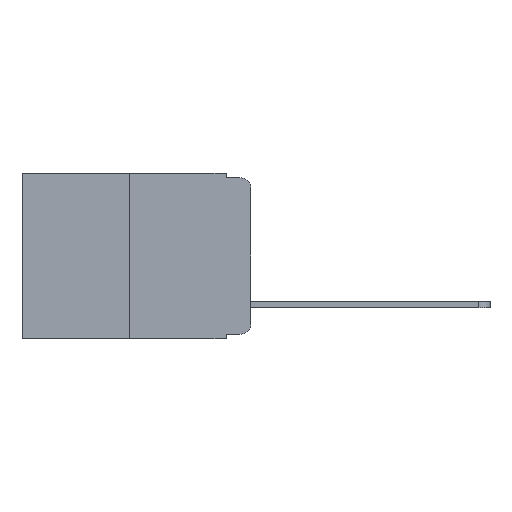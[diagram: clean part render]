
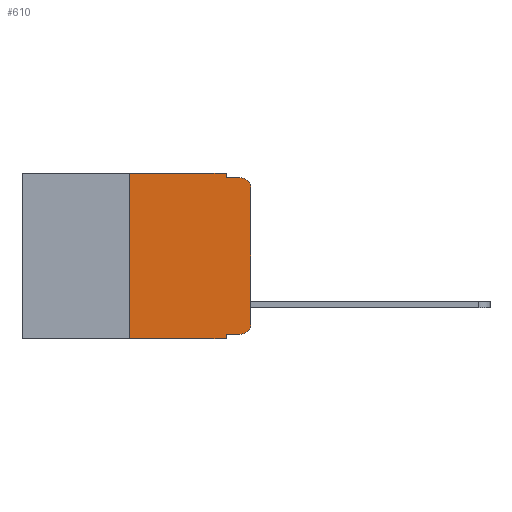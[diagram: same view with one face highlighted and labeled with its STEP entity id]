
A CAD part, left-side view. The second image highlights one B-rep face of the part: STEP entity #610.
In plain terms, the highlighted planar face has unit normal (-1, 0, 0).
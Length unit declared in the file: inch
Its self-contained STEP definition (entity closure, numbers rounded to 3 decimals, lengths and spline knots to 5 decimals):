
#143 = VERTEX_POINT ( 'NONE', #9389 ) ;
#241 = CARTESIAN_POINT ( 'NONE',  ( 0., 0.051, 0. ) ) ;
#284 = ORIENTED_EDGE ( 'NONE', *, *, #2498, .F. ) ;
#610 = ADVANCED_FACE ( 'NONE', ( #7530 ), #2642, .F. ) ;
#1050 = VERTEX_POINT ( 'NONE', #1367 ) ;
#1134 = EDGE_CURVE ( 'NONE', #5379, #143, #9879, .T. ) ;
#1167 = CARTESIAN_POINT ( 'NONE',  ( 0., 0.02, -0.03 ) ) ;
#1315 = DIRECTION ( 'NONE',  ( 0., 0., -1. ) ) ;
#1367 = CARTESIAN_POINT ( 'NONE',  ( 0., 0.051, -0.333 ) ) ;
#1408 = EDGE_CURVE ( 'NONE', #9601, #5036, #2824, .T. ) ;
#1498 = CARTESIAN_POINT ( 'NONE',  ( 0., 0., 0. ) ) ;
#1551 = EDGE_CURVE ( 'NONE', #2093, #10796, #10320, .T. ) ;
#1696 = CARTESIAN_POINT ( 'NONE',  ( 0., 0.473, 0. ) ) ;
#1870 = LINE ( 'NONE', #1498, #2463 ) ;
#1888 = VECTOR ( 'NONE', #8993, 39.37008 ) ;
#2073 = ORIENTED_EDGE ( 'NONE', *, *, #2184, .F. ) ;
#2093 = VERTEX_POINT ( 'NONE', #9987 ) ;
#2184 = EDGE_CURVE ( 'NONE', #9601, #8978, #5876, .T. ) ;
#2463 = VECTOR ( 'NONE', #3433, 39.37008 ) ;
#2498 = EDGE_CURVE ( 'NONE', #10796, #9502, #9255, .T. ) ;
#2527 = VECTOR ( 'NONE', #11309, 39.37008 ) ;
#2642 = PLANE ( 'NONE',  #5559 ) ;
#2744 = ORIENTED_EDGE ( 'NONE', *, *, #3947, .T. ) ;
#2749 = LINE ( 'NONE', #4065, #4204 ) ;
#2762 = CARTESIAN_POINT ( 'NONE',  ( 0., 0.25, -0.343 ) ) ;
#2796 = CARTESIAN_POINT ( 'NONE',  ( 0., 0.02, -0.01 ) ) ;
#2824 = LINE ( 'NONE', #5761, #2527 ) ;
#3064 = CIRCLE ( 'NONE', #4693, 0.02 ) ;
#3115 = ORIENTED_EDGE ( 'NONE', *, *, #6424, .F. ) ;
#3316 = CARTESIAN_POINT ( 'NONE',  ( 0., 0., -0.03 ) ) ;
#3433 = DIRECTION ( 'NONE',  ( 0., 0., 1. ) ) ;
#3551 = AXIS2_PLACEMENT_3D ( 'NONE', #6342, #9984, #4507 ) ;
#3702 = CARTESIAN_POINT ( 'NONE',  ( 0., 0.25, 0. ) ) ;
#3947 = EDGE_CURVE ( 'NONE', #1050, #5379, #6861, .T. ) ;
#4065 = CARTESIAN_POINT ( 'NONE',  ( 0., 0.051, 0. ) ) ;
#4204 = VECTOR ( 'NONE', #5997, 39.37008 ) ;
#4219 = DIRECTION ( 'NONE',  ( 0., -1., 0. ) ) ;
#4507 = DIRECTION ( 'NONE',  ( 0., 0., -1. ) ) ;
#4563 = DIRECTION ( 'NONE',  ( 0., 0., -1. ) ) ;
#4693 = AXIS2_PLACEMENT_3D ( 'NONE', #1167, #11409, #7634 ) ;
#4730 = CARTESIAN_POINT ( 'NONE',  ( 0., 0.051, -0.01 ) ) ;
#4740 = ORIENTED_EDGE ( 'NONE', *, *, #6006, .F. ) ;
#5036 = VERTEX_POINT ( 'NONE', #7479 ) ;
#5135 = ORIENTED_EDGE ( 'NONE', *, *, #1408, .T. ) ;
#5379 = VERTEX_POINT ( 'NONE', #8290 ) ;
#5511 = DIRECTION ( 'NONE',  ( 1., 0., 0. ) ) ;
#5559 = AXIS2_PLACEMENT_3D ( 'NONE', #1696, #5511, #4563 ) ;
#5761 = CARTESIAN_POINT ( 'NONE',  ( 0., 0.473, -0.343 ) ) ;
#5827 = LINE ( 'NONE', #9181, #7737 ) ;
#5876 = LINE ( 'NONE', #3702, #11315 ) ;
#5997 = DIRECTION ( 'NONE',  ( 0., 0., -1. ) ) ;
#6006 = EDGE_CURVE ( 'NONE', #8978, #2093, #5827, .T. ) ;
#6198 = EDGE_CURVE ( 'NONE', #143, #9372, #1870, .T. ) ;
#6342 = CARTESIAN_POINT ( 'NONE',  ( 0., 0.02, -0.313 ) ) ;
#6424 = EDGE_CURVE ( 'NONE', #1050, #5036, #2749, .T. ) ;
#6505 = DIRECTION ( 'NONE',  ( 0., 0., 1. ) ) ;
#6861 = LINE ( 'NONE', #11003, #1888 ) ;
#7128 = CARTESIAN_POINT ( 'NONE',  ( 0., 0.051, -0.01 ) ) ;
#7479 = CARTESIAN_POINT ( 'NONE',  ( 0., 0.051, -0.343 ) ) ;
#7530 = FACE_OUTER_BOUND ( 'NONE', #9811, .T. ) ;
#7634 = DIRECTION ( 'NONE',  ( 0., 0., -1. ) ) ;
#7737 = VECTOR ( 'NONE', #8162, 39.37008 ) ;
#8162 = DIRECTION ( 'NONE',  ( 0., -1., 0. ) ) ;
#8290 = CARTESIAN_POINT ( 'NONE',  ( 0., 0.02, -0.333 ) ) ;
#8313 = ORIENTED_EDGE ( 'NONE', *, *, #11482, .T. ) ;
#8820 = VECTOR ( 'NONE', #4219, 39.37008 ) ;
#8825 = CARTESIAN_POINT ( 'NONE',  ( 0., 0.25, 0. ) ) ;
#8955 = ORIENTED_EDGE ( 'NONE', *, *, #1134, .T. ) ;
#8978 = VERTEX_POINT ( 'NONE', #8825 ) ;
#8993 = DIRECTION ( 'NONE',  ( 0., -1., 0. ) ) ;
#9181 = CARTESIAN_POINT ( 'NONE',  ( 0., 0.473, 0. ) ) ;
#9255 = LINE ( 'NONE', #7128, #8820 ) ;
#9372 = VERTEX_POINT ( 'NONE', #3316 ) ;
#9389 = CARTESIAN_POINT ( 'NONE',  ( 0., 0., -0.313 ) ) ;
#9502 = VERTEX_POINT ( 'NONE', #2796 ) ;
#9601 = VERTEX_POINT ( 'NONE', #2762 ) ;
#9811 = EDGE_LOOP ( 'NONE', ( #11394, #8313, #284, #11753, #4740, #2073, #5135, #3115, #2744, #8955 ) ) ;
#9879 = CIRCLE ( 'NONE', #3551, 0.02 ) ;
#9984 = DIRECTION ( 'NONE',  ( -1., 0., 0. ) ) ;
#9987 = CARTESIAN_POINT ( 'NONE',  ( 0., 0.051, 0. ) ) ;
#10320 = LINE ( 'NONE', #241, #11930 ) ;
#10796 = VERTEX_POINT ( 'NONE', #4730 ) ;
#11003 = CARTESIAN_POINT ( 'NONE',  ( 0., 0.051, -0.333 ) ) ;
#11309 = DIRECTION ( 'NONE',  ( 0., -1., 0. ) ) ;
#11315 = VECTOR ( 'NONE', #6505, 39.37008 ) ;
#11394 = ORIENTED_EDGE ( 'NONE', *, *, #6198, .T. ) ;
#11409 = DIRECTION ( 'NONE',  ( -1., 0., 0. ) ) ;
#11482 = EDGE_CURVE ( 'NONE', #9372, #9502, #3064, .T. ) ;
#11753 = ORIENTED_EDGE ( 'NONE', *, *, #1551, .F. ) ;
#11930 = VECTOR ( 'NONE', #1315, 39.37008 ) ;
